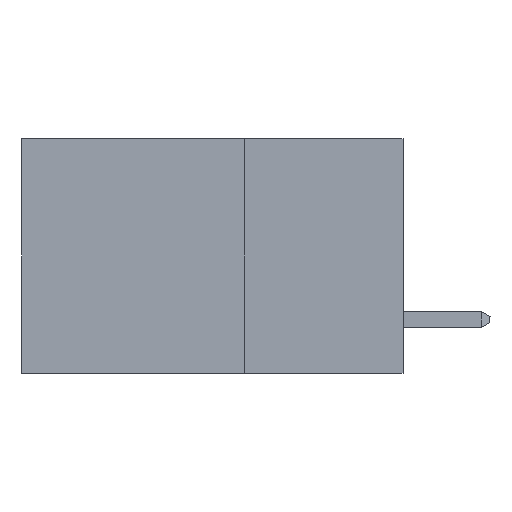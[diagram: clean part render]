
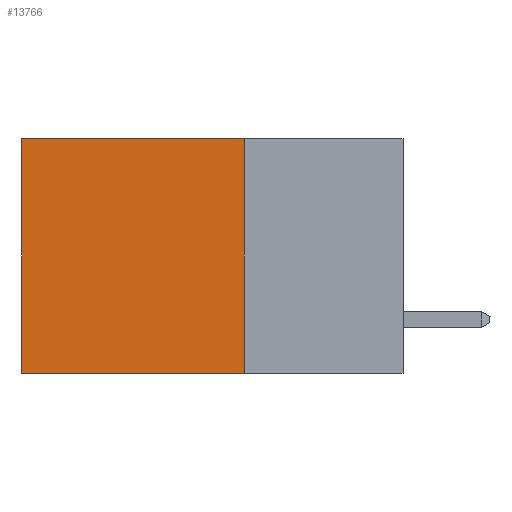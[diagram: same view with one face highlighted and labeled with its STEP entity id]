
A CAD part, left-side view. The second image highlights one B-rep face of the part: STEP entity #13766.
In plain terms, the highlighted planar face has unit normal (-1, 0, 0).
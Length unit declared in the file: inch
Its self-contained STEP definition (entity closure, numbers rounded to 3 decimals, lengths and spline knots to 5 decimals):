
#446 = EDGE_CURVE ( 'NONE', #17042, #6184, #22373, .T. ) ;
#756 = CARTESIAN_POINT ( 'NONE',  ( 0.2875, 0.25, 0. ) ) ;
#2095 = DIRECTION ( 'NONE',  ( 0., 1., 0. ) ) ;
#2250 = DIRECTION ( 'NONE',  ( 1., 0., 0. ) ) ;
#2448 = VECTOR ( 'NONE', #23081, 39.37008 ) ;
#2495 = CARTESIAN_POINT ( 'NONE',  ( 0.2875, 0.25, -0.37 ) ) ;
#3919 = LINE ( 'NONE', #18743, #16223 ) ;
#4083 = DIRECTION ( 'NONE',  ( 0., 0., -1. ) ) ;
#5504 = DIRECTION ( 'NONE',  ( 0., 0., -1. ) ) ;
#6034 = PLANE ( 'NONE',  #21842 ) ;
#6184 = VERTEX_POINT ( 'NONE', #2495 ) ;
#6216 = ORIENTED_EDGE ( 'NONE', *, *, #21693, .T. ) ;
#7742 = VECTOR ( 'NONE', #5504, 39.37008 ) ;
#8453 = CARTESIAN_POINT ( 'NONE',  ( 0.2875, 0.6, 0. ) ) ;
#8947 = EDGE_CURVE ( 'NONE', #6184, #22739, #3919, .T. ) ;
#10333 = CARTESIAN_POINT ( 'NONE',  ( 0.2875, 0.6, 0. ) ) ;
#10936 = VECTOR ( 'NONE', #17539, 39.37008 ) ;
#12663 = EDGE_LOOP ( 'NONE', ( #21158, #21474, #16856, #6216 ) ) ;
#13766 = ADVANCED_FACE ( 'NONE', ( #16956 ), #6034, .F. ) ;
#14717 = CARTESIAN_POINT ( 'NONE',  ( 0.2875, 0.6, -0.37 ) ) ;
#14939 = CARTESIAN_POINT ( 'NONE',  ( 0.2875, 0.25, 0. ) ) ;
#15239 = VERTEX_POINT ( 'NONE', #8453 ) ;
#15484 = CARTESIAN_POINT ( 'NONE',  ( 0.2875, 0.25, 0. ) ) ;
#16223 = VECTOR ( 'NONE', #2095, 39.37008 ) ;
#16856 = ORIENTED_EDGE ( 'NONE', *, *, #446, .F. ) ;
#16956 = FACE_OUTER_BOUND ( 'NONE', #12663, .T. ) ;
#17042 = VERTEX_POINT ( 'NONE', #14939 ) ;
#17539 = DIRECTION ( 'NONE',  ( 0., 1., 0. ) ) ;
#18743 = CARTESIAN_POINT ( 'NONE',  ( 0.2875, 0.25, -0.37 ) ) ;
#18857 = CARTESIAN_POINT ( 'NONE',  ( 0.2875, 0.25, 0. ) ) ;
#19346 = LINE ( 'NONE', #756, #10936 ) ;
#21158 = ORIENTED_EDGE ( 'NONE', *, *, #23380, .T. ) ;
#21474 = ORIENTED_EDGE ( 'NONE', *, *, #8947, .F. ) ;
#21693 = EDGE_CURVE ( 'NONE', #17042, #15239, #19346, .T. ) ;
#21842 = AXIS2_PLACEMENT_3D ( 'NONE', #15484, #2250, #4083 ) ;
#22373 = LINE ( 'NONE', #18857, #7742 ) ;
#22739 = VERTEX_POINT ( 'NONE', #14717 ) ;
#22967 = LINE ( 'NONE', #10333, #2448 ) ;
#23081 = DIRECTION ( 'NONE',  ( 0., 0., -1. ) ) ;
#23380 = EDGE_CURVE ( 'NONE', #15239, #22739, #22967, .T. ) ;
